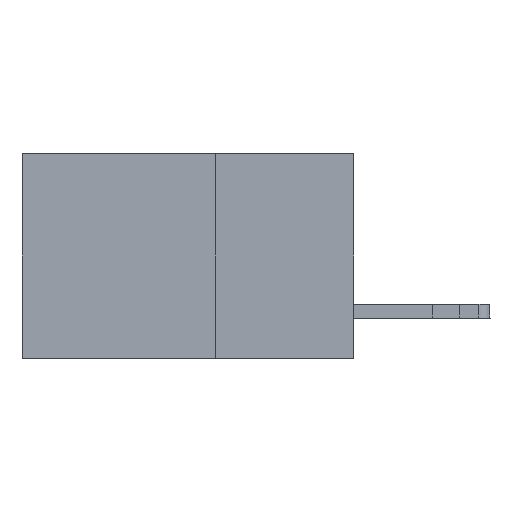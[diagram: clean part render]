
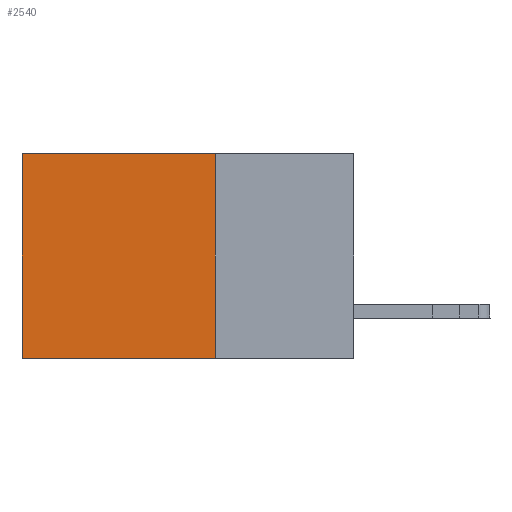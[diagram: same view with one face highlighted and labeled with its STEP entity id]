
A CAD part, left-side view. The second image highlights one B-rep face of the part: STEP entity #2540.
In plain terms, the highlighted planar face has unit normal (-1, 0, 0).
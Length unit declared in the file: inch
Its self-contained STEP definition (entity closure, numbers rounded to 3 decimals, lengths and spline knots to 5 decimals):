
#167 = VERTEX_POINT ( 'NONE', #14078 ) ;
#599 = DIRECTION ( 'NONE',  ( 0., 0., -1. ) ) ;
#929 = FACE_OUTER_BOUND ( 'NONE', #16139, .T. ) ;
#1939 = EDGE_CURVE ( 'NONE', #4283, #6157, #17527, .T. ) ;
#2095 = EDGE_CURVE ( 'NONE', #12047, #167, #3041, .T. ) ;
#2540 = ADVANCED_FACE ( 'NONE', ( #929 ), #4992, .F. ) ;
#3041 = LINE ( 'NONE', #16818, #14899 ) ;
#4006 = DIRECTION ( 'NONE',  ( 0., 0., -1. ) ) ;
#4111 = DIRECTION ( 'NONE',  ( 0., 0., -1. ) ) ;
#4186 = VECTOR ( 'NONE', #4111, 39.37008 ) ;
#4283 = VERTEX_POINT ( 'NONE', #14391 ) ;
#4992 = PLANE ( 'NONE',  #17462 ) ;
#6157 = VERTEX_POINT ( 'NONE', #10593 ) ;
#6623 = EDGE_CURVE ( 'NONE', #12047, #4283, #17417, .T. ) ;
#6665 = DIRECTION ( 'NONE',  ( 0., 1., 0. ) ) ;
#8106 = ORIENTED_EDGE ( 'NONE', *, *, #1939, .F. ) ;
#8353 = CARTESIAN_POINT ( 'NONE',  ( 0.2875, 0.25, -0.37 ) ) ;
#8623 = ORIENTED_EDGE ( 'NONE', *, *, #6623, .F. ) ;
#8953 = ORIENTED_EDGE ( 'NONE', *, *, #10131, .T. ) ;
#9099 = LINE ( 'NONE', #13293, #17516 ) ;
#9176 = DIRECTION ( 'NONE',  ( 0., 1., 0. ) ) ;
#9788 = CARTESIAN_POINT ( 'NONE',  ( 0.2875, 0.25, 0. ) ) ;
#10131 = EDGE_CURVE ( 'NONE', #167, #6157, #9099, .T. ) ;
#10593 = CARTESIAN_POINT ( 'NONE',  ( 0.2875, 0.6, -0.37 ) ) ;
#12047 = VERTEX_POINT ( 'NONE', #13372 ) ;
#13293 = CARTESIAN_POINT ( 'NONE',  ( 0.2875, 0.6, 0. ) ) ;
#13372 = CARTESIAN_POINT ( 'NONE',  ( 0.2875, 0.25, 0. ) ) ;
#14078 = CARTESIAN_POINT ( 'NONE',  ( 0.2875, 0.6, 0. ) ) ;
#14391 = CARTESIAN_POINT ( 'NONE',  ( 0.2875, 0.25, -0.37 ) ) ;
#14899 = VECTOR ( 'NONE', #9176, 39.37008 ) ;
#15348 = ORIENTED_EDGE ( 'NONE', *, *, #2095, .T. ) ;
#16139 = EDGE_LOOP ( 'NONE', ( #8953, #8106, #8623, #15348 ) ) ;
#16818 = CARTESIAN_POINT ( 'NONE',  ( 0.2875, 0.25, 0. ) ) ;
#17300 = DIRECTION ( 'NONE',  ( 1., 0., 0. ) ) ;
#17417 = LINE ( 'NONE', #18980, #4186 ) ;
#17462 = AXIS2_PLACEMENT_3D ( 'NONE', #9788, #17300, #599 ) ;
#17516 = VECTOR ( 'NONE', #4006, 39.37008 ) ;
#17527 = LINE ( 'NONE', #8353, #17760 ) ;
#17760 = VECTOR ( 'NONE', #6665, 39.37008 ) ;
#18980 = CARTESIAN_POINT ( 'NONE',  ( 0.2875, 0.25, 0. ) ) ;
